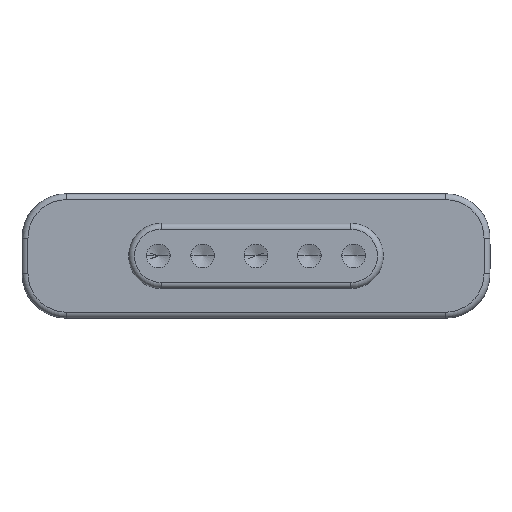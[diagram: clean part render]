
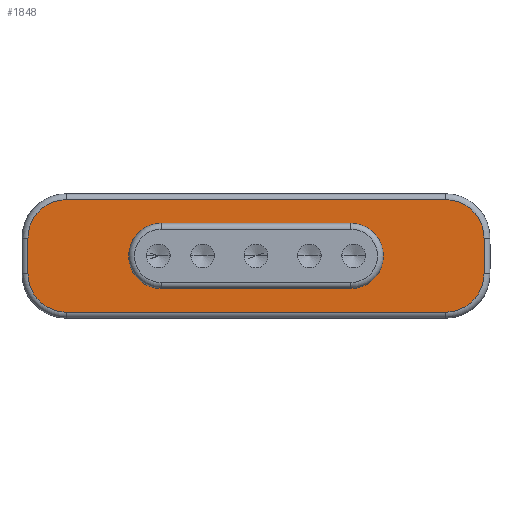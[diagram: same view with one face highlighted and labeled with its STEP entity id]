
A CAD part, top view. The second image highlights one B-rep face of the part: STEP entity #1848.
In plain terms, the highlighted planar face has unit normal (0, 0, 1).
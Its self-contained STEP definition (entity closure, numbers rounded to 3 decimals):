
#11 = EDGE_CURVE ( 'NONE', #2754, #489, #1381, .T. ) ;
#57 = DIRECTION ( 'NONE',  ( 1., 0., 0. ) ) ;
#86 = EDGE_CURVE ( 'NONE', #2574, #954, #3377, .T. ) ;
#95 = CARTESIAN_POINT ( 'NONE',  ( 3.2, 0., -0.15 ) ) ;
#152 = AXIS2_PLACEMENT_3D ( 'NONE', #2600, #872, #2313 ) ;
#170 = VERTEX_POINT ( 'NONE', #4408 ) ;
#205 = VERTEX_POINT ( 'NONE', #3366 ) ;
#230 = VECTOR ( 'NONE', #749, 1000. ) ;
#240 = DIRECTION ( 'NONE',  ( 0., 1., 0. ) ) ;
#248 = VERTEX_POINT ( 'NONE', #4006 ) ;
#293 = CARTESIAN_POINT ( 'NONE',  ( -3.2, 0., -0.15 ) ) ;
#319 = EDGE_CURVE ( 'NONE', #2754, #3194, #746, .T. ) ;
#325 = ORIENTED_EDGE ( 'NONE', *, *, #2633, .T. ) ;
#374 = VECTOR ( 'NONE', #1142, 1000. ) ;
#380 = CARTESIAN_POINT ( 'NONE',  ( 3.2, -1.1, -0.15 ) ) ;
#415 = PLANE ( 'NONE',  #966 ) ;
#489 = VERTEX_POINT ( 'NONE', #3197 ) ;
#571 = CIRCLE ( 'NONE', #4457, 1.1 ) ;
#609 = VERTEX_POINT ( 'NONE', #2906 ) ;
#638 = ORIENTED_EDGE ( 'NONE', *, *, #319, .F. ) ;
#746 = CIRCLE ( 'NONE', #3801, 1.3 ) ;
#749 = DIRECTION ( 'NONE',  ( 1., 0., 0. ) ) ;
#848 = DIRECTION ( 'NONE',  ( -1., 0., 0. ) ) ;
#872 = DIRECTION ( 'NONE',  ( 0., 0., 1. ) ) ;
#954 = VERTEX_POINT ( 'NONE', #1365 ) ;
#966 = AXIS2_PLACEMENT_3D ( 'NONE', #1873, #3336, #57 ) ;
#1045 = CARTESIAN_POINT ( 'NONE',  ( -3.2, 1.1, -0.15 ) ) ;
#1064 = EDGE_CURVE ( 'NONE', #3079, #248, #2881, .T. ) ;
#1066 = CARTESIAN_POINT ( 'NONE',  ( 6.4, -0.6, -0.15 ) ) ;
#1094 = ORIENTED_EDGE ( 'NONE', *, *, #11, .T. ) ;
#1142 = DIRECTION ( 'NONE',  ( -1., 0., 0. ) ) ;
#1154 = ORIENTED_EDGE ( 'NONE', *, *, #2024, .F. ) ;
#1201 = DIRECTION ( 'NONE',  ( 0., -1., 0. ) ) ;
#1229 = CARTESIAN_POINT ( 'NONE',  ( -6.4, 0.6, -0.15 ) ) ;
#1240 = EDGE_CURVE ( 'NONE', #2574, #1638, #1391, .T. ) ;
#1253 = ORIENTED_EDGE ( 'NONE', *, *, #2525, .T. ) ;
#1270 = DIRECTION ( 'NONE',  ( 0., 1., 0. ) ) ;
#1292 = AXIS2_PLACEMENT_3D ( 'NONE', #4543, #2792, #1270 ) ;
#1334 = LINE ( 'NONE', #1360, #2057 ) ;
#1352 = AXIS2_PLACEMENT_3D ( 'NONE', #2353, #3832, #1201 ) ;
#1360 = CARTESIAN_POINT ( 'NONE',  ( 6.4, 1.9, -0.15 ) ) ;
#1365 = CARTESIAN_POINT ( 'NONE',  ( 6.4, -1.9, -0.15 ) ) ;
#1381 = LINE ( 'NONE', #2889, #2088 ) ;
#1391 = LINE ( 'NONE', #2392, #4167 ) ;
#1551 = DIRECTION ( 'NONE',  ( 0., 0., 1. ) ) ;
#1638 = VERTEX_POINT ( 'NONE', #2841 ) ;
#1835 = DIRECTION ( 'NONE',  ( 1., 0., 0. ) ) ;
#1848 = ADVANCED_FACE ( 'NONE', ( #4077, #3693 ), #415, .T. ) ;
#1851 = ORIENTED_EDGE ( 'NONE', *, *, #3363, .F. ) ;
#1873 = CARTESIAN_POINT ( 'NONE',  ( 0., 0., -0.15 ) ) ;
#1883 = CARTESIAN_POINT ( 'NONE',  ( -7.7, 0.6, -0.15 ) ) ;
#1902 = EDGE_CURVE ( 'NONE', #3133, #489, #4176, .T. ) ;
#1923 = AXIS2_PLACEMENT_3D ( 'NONE', #1066, #4672, #3508 ) ;
#2024 = EDGE_CURVE ( 'NONE', #3079, #205, #2810, .T. ) ;
#2057 = VECTOR ( 'NONE', #3519, 1000. ) ;
#2062 = CIRCLE ( 'NONE', #152, 1.1 ) ;
#2088 = VECTOR ( 'NONE', #2819, 1000. ) ;
#2109 = CARTESIAN_POINT ( 'NONE',  ( 7.7, -0.6, -0.15 ) ) ;
#2247 = CARTESIAN_POINT ( 'NONE',  ( -6.4, 1.9, -0.15 ) ) ;
#2252 = CARTESIAN_POINT ( 'NONE',  ( -6.4, -1.9, -0.15 ) ) ;
#2298 = CIRCLE ( 'NONE', #1292, 1.3 ) ;
#2313 = DIRECTION ( 'NONE',  ( 1., 0., 0. ) ) ;
#2353 = CARTESIAN_POINT ( 'NONE',  ( -6.4, -0.6, -0.15 ) ) ;
#2392 = CARTESIAN_POINT ( 'NONE',  ( 7.7, -0.6, -0.15 ) ) ;
#2505 = AXIS2_PLACEMENT_3D ( 'NONE', #293, #2882, #2858 ) ;
#2514 = CARTESIAN_POINT ( 'NONE',  ( -3.2, 1.1, -0.15 ) ) ;
#2525 = EDGE_CURVE ( 'NONE', #170, #3194, #1334, .T. ) ;
#2536 = ORIENTED_EDGE ( 'NONE', *, *, #1064, .T. ) ;
#2558 = LINE ( 'NONE', #380, #374 ) ;
#2574 = VERTEX_POINT ( 'NONE', #2109 ) ;
#2600 = CARTESIAN_POINT ( 'NONE',  ( 3.2, 0., -0.15 ) ) ;
#2633 = EDGE_CURVE ( 'NONE', #3133, #954, #3616, .T. ) ;
#2643 = EDGE_CURVE ( 'NONE', #609, #205, #2558, .T. ) ;
#2754 = VERTEX_POINT ( 'NONE', #1883 ) ;
#2760 = ORIENTED_EDGE ( 'NONE', *, *, #3840, .F. ) ;
#2780 = VERTEX_POINT ( 'NONE', #3375 ) ;
#2792 = DIRECTION ( 'NONE',  ( 0., 0., -1. ) ) ;
#2810 = CIRCLE ( 'NONE', #2505, 1.1 ) ;
#2819 = DIRECTION ( 'NONE',  ( 0., -1., 0. ) ) ;
#2841 = CARTESIAN_POINT ( 'NONE',  ( 7.7, 0.6, -0.15 ) ) ;
#2858 = DIRECTION ( 'NONE',  ( -1., 0., 0. ) ) ;
#2881 = LINE ( 'NONE', #2514, #230 ) ;
#2882 = DIRECTION ( 'NONE',  ( 0., 0., 1. ) ) ;
#2889 = CARTESIAN_POINT ( 'NONE',  ( -7.7, 0.6, -0.15 ) ) ;
#2898 = ORIENTED_EDGE ( 'NONE', *, *, #86, .F. ) ;
#2906 = CARTESIAN_POINT ( 'NONE',  ( 3.2, -1.1, -0.15 ) ) ;
#3013 = DIRECTION ( 'NONE',  ( 1., 0., 0. ) ) ;
#3026 = ORIENTED_EDGE ( 'NONE', *, *, #1240, .T. ) ;
#3078 = EDGE_LOOP ( 'NONE', ( #638, #1094, #3639, #325, #2898, #3026, #1851, #1253 ) ) ;
#3079 = VERTEX_POINT ( 'NONE', #1045 ) ;
#3133 = VERTEX_POINT ( 'NONE', #3747 ) ;
#3139 = EDGE_CURVE ( 'NONE', #609, #2780, #2062, .T. ) ;
#3194 = VERTEX_POINT ( 'NONE', #2247 ) ;
#3197 = CARTESIAN_POINT ( 'NONE',  ( -7.7, -0.6, -0.15 ) ) ;
#3336 = DIRECTION ( 'NONE',  ( 0., 0., 1. ) ) ;
#3363 = EDGE_CURVE ( 'NONE', #170, #1638, #2298, .T. ) ;
#3366 = CARTESIAN_POINT ( 'NONE',  ( -3.2, -1.1, -0.15 ) ) ;
#3375 = CARTESIAN_POINT ( 'NONE',  ( 4.3, 0., -0.15 ) ) ;
#3377 = CIRCLE ( 'NONE', #1923, 1.3 ) ;
#3488 = EDGE_LOOP ( 'NONE', ( #4612, #4721, #1154, #2536, #2760 ) ) ;
#3508 = DIRECTION ( 'NONE',  ( 1., 0., 0. ) ) ;
#3510 = VECTOR ( 'NONE', #1835, 1000. ) ;
#3519 = DIRECTION ( 'NONE',  ( -1., 0., 0. ) ) ;
#3616 = LINE ( 'NONE', #2252, #3510 ) ;
#3639 = ORIENTED_EDGE ( 'NONE', *, *, #1902, .F. ) ;
#3693 = FACE_OUTER_BOUND ( 'NONE', #3078, .T. ) ;
#3747 = CARTESIAN_POINT ( 'NONE',  ( -6.4, -1.9, -0.15 ) ) ;
#3801 = AXIS2_PLACEMENT_3D ( 'NONE', #1229, #4518, #848 ) ;
#3832 = DIRECTION ( 'NONE',  ( 0., 0., -1. ) ) ;
#3840 = EDGE_CURVE ( 'NONE', #2780, #248, #571, .T. ) ;
#4006 = CARTESIAN_POINT ( 'NONE',  ( 3.2, 1.1, -0.15 ) ) ;
#4077 = FACE_BOUND ( 'NONE', #3488, .T. ) ;
#4167 = VECTOR ( 'NONE', #240, 1000. ) ;
#4176 = CIRCLE ( 'NONE', #1352, 1.3 ) ;
#4408 = CARTESIAN_POINT ( 'NONE',  ( 6.4, 1.9, -0.15 ) ) ;
#4457 = AXIS2_PLACEMENT_3D ( 'NONE', #95, #1551, #3013 ) ;
#4518 = DIRECTION ( 'NONE',  ( 0., 0., -1. ) ) ;
#4543 = CARTESIAN_POINT ( 'NONE',  ( 6.4, 0.6, -0.15 ) ) ;
#4612 = ORIENTED_EDGE ( 'NONE', *, *, #3139, .F. ) ;
#4672 = DIRECTION ( 'NONE',  ( 0., 0., -1. ) ) ;
#4721 = ORIENTED_EDGE ( 'NONE', *, *, #2643, .T. ) ;
